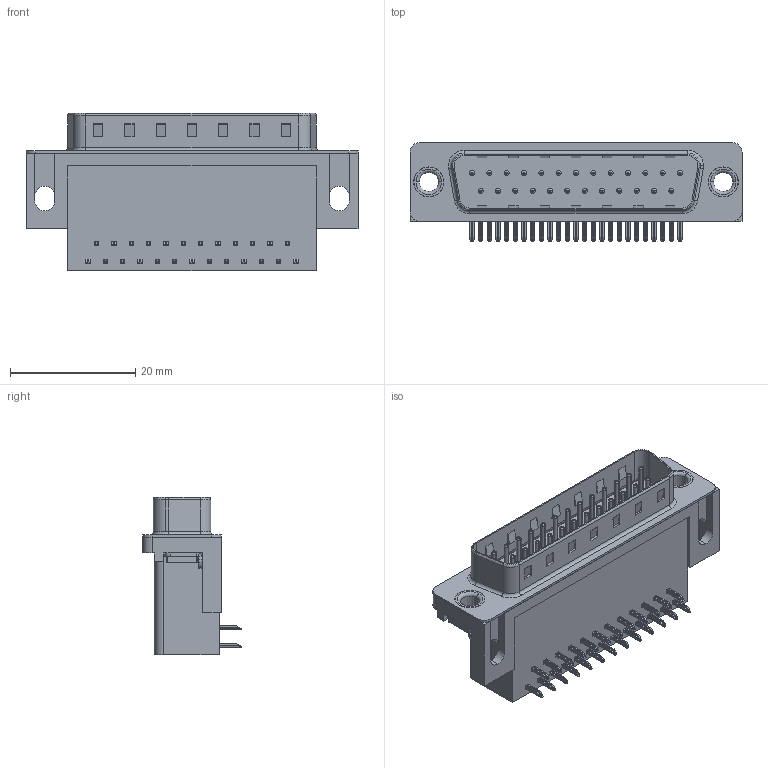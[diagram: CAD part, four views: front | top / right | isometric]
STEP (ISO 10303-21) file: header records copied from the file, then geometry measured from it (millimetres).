
FILE_DESCRIPTION (( 'STEP AP203' ), '1' );
FILE_NAME ('625-025-362-501.STEP', '2018-11-06T02:34:58', ( '' ), ( '' ), 'SwSTEP 2.0', 'SolidWorks 2016', '' );
FILE_SCHEMA (( 'CONFIG_CONTROL_DESIGN' ));
Length unit declared in the file: millimetre
Products named in the file (7): 625 Non Board Mount; 625 Thru Hole Rivet; 625-025-362-501; 625 Housing_25 Socket; 625 Shell_25 Socket; 625 Contact Bottom; 625 Contact Top
Assembly tree (31 placements, depth 2):
  625-025-362-501
    625 Housing_25 Socket
    625 Shell_25 Socket
    625 Contact Bottom  x12
    625 Contact Top  x13
    625 Non Board Mount  x2
    625 Thru Hole Rivet  x2
Bounding box: 53.04 x 15.73 x 25.16 mm (x, y, z)
Volume: 9124.5 mm3; surface area: 8704.2 mm2
Topology: 31 solids, 31 shells, 2223 faces, 5495 edges, 3391 vertices
Faces by surface type: plane 1407, cylinder 639, torus 177
Entity records: 20361 total; most frequent: DIRECTION 3336, CARTESIAN_POINT 3291, ORIENTED_EDGE 3160, EDGE_CURVE 1580, VECTOR 1140, LINE 1140, AXIS2_PLACEMENT_3D 1098, VERTEX_POINT 1013
